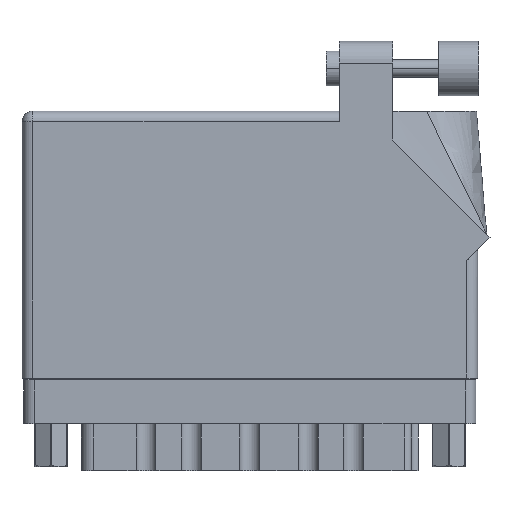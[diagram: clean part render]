
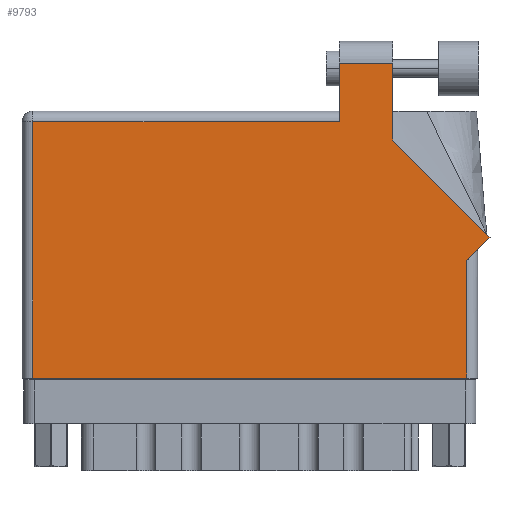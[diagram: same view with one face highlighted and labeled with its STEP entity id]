
A CAD part, front view. The second image highlights one B-rep face of the part: STEP entity #9793.
In plain terms, the highlighted face is planar.
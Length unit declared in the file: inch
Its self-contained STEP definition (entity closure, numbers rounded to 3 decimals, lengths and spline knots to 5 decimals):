
#339 = EDGE_CURVE ( 'NONE', #10485, #43581, #3423, .T. ) ;
#1990 = VERTEX_POINT ( 'NONE', #50898 ) ;
#2652 = CARTESIAN_POINT ( 'NONE',  ( 2.55, 0.675, 0. ) ) ;
#2788 = CARTESIAN_POINT ( 'NONE',  ( 2.68271, 0.80771, 0. ) ) ;
#3423 = LINE ( 'NONE', #22628, #28336 ) ;
#4869 = DIRECTION ( 'NONE',  ( 0., 1., 0. ) ) ;
#5986 = EDGE_CURVE ( 'NONE', #24299, #54785, #29102, .T. ) ;
#6192 = VECTOR ( 'NONE', #15545, 39.37008 ) ;
#6231 = CARTESIAN_POINT ( 'NONE',  ( 0.062, 0., 0. ) ) ;
#6344 = CARTESIAN_POINT ( 'NONE',  ( 2.126, 1.805, 0. ) ) ;
#7420 = LINE ( 'NONE', #25991, #21301 ) ;
#8194 = CARTESIAN_POINT ( 'NONE',  ( 2.55, 0., 0. ) ) ;
#9665 = EDGE_CURVE ( 'NONE', #24457, #12983, #50404, .T. ) ;
#9793 = ADVANCED_FACE ( 'NONE', ( #14433 ), #18517, .F. ) ;
#10485 = VERTEX_POINT ( 'NONE', #60340 ) ;
#10664 = ORIENTED_EDGE ( 'NONE', *, *, #339, .T. ) ;
#12126 = ORIENTED_EDGE ( 'NONE', *, *, #16217, .T. ) ;
#12679 = ORIENTED_EDGE ( 'NONE', *, *, #15060, .T. ) ;
#12983 = VERTEX_POINT ( 'NONE', #47654 ) ;
#14296 = LINE ( 'NONE', #19327, #6192 ) ;
#14376 = ORIENTED_EDGE ( 'NONE', *, *, #9665, .T. ) ;
#14433 = FACE_OUTER_BOUND ( 'NONE', #40207, .T. ) ;
#14602 = CARTESIAN_POINT ( 'NONE',  ( 1.819, 1.805, 0. ) ) ;
#14739 = DIRECTION ( 'NONE',  ( -0.707, 0.707, 0. ) ) ;
#15060 = EDGE_CURVE ( 'NONE', #43581, #24299, #20052, .T. ) ;
#15545 = DIRECTION ( 'NONE',  ( 0., 1., 0. ) ) ;
#16217 = EDGE_CURVE ( 'NONE', #1990, #30200, #33837, .T. ) ;
#17422 = EDGE_CURVE ( 'NONE', #54785, #24457, #42731, .T. ) ;
#18517 = PLANE ( 'NONE',  #32295 ) ;
#19327 = CARTESIAN_POINT ( 'NONE',  ( 2.126, 1.36442, 0. ) ) ;
#19530 = CARTESIAN_POINT ( 'NONE',  ( 2.68271, 0.80771, 0. ) ) ;
#20052 = LINE ( 'NONE', #34207, #56727 ) ;
#21301 = VECTOR ( 'NONE', #45898, 39.37008 ) ;
#22628 = CARTESIAN_POINT ( 'NONE',  ( 0.062, 0., 0. ) ) ;
#23240 = VECTOR ( 'NONE', #14739, 39.37008 ) ;
#23478 = DIRECTION ( 'NONE',  ( 0., -1., 0. ) ) ;
#24299 = VERTEX_POINT ( 'NONE', #8194 ) ;
#24457 = VERTEX_POINT ( 'NONE', #19530 ) ;
#25991 = CARTESIAN_POINT ( 'NONE',  ( 0., 1.468, 0. ) ) ;
#27640 = ORIENTED_EDGE ( 'NONE', *, *, #17422, .T. ) ;
#28336 = VECTOR ( 'NONE', #56695, 39.37008 ) ;
#29102 = LINE ( 'NONE', #51867, #45585 ) ;
#30200 = VERTEX_POINT ( 'NONE', #54878 ) ;
#31671 = DIRECTION ( 'NONE',  ( 0.707, 0.707, 0. ) ) ;
#32295 = AXIS2_PLACEMENT_3D ( 'NONE', #33605, #38680, #52894 ) ;
#32795 = EDGE_CURVE ( 'NONE', #30200, #10485, #7420, .T. ) ;
#33204 = CARTESIAN_POINT ( 'NONE',  ( 1.819, 1.53, 0. ) ) ;
#33605 = CARTESIAN_POINT ( 'NONE',  ( 0., 1.53, 0. ) ) ;
#33779 = DIRECTION ( 'NONE',  ( -1., 0., 0. ) ) ;
#33837 = LINE ( 'NONE', #33204, #48036 ) ;
#34207 = CARTESIAN_POINT ( 'NONE',  ( 0., 0., 0. ) ) ;
#37326 = ORIENTED_EDGE ( 'NONE', *, *, #60133, .T. ) ;
#38030 = DIRECTION ( 'NONE',  ( 1., 0., 0. ) ) ;
#38680 = DIRECTION ( 'NONE',  ( 0., 0., -1. ) ) ;
#40207 = EDGE_LOOP ( 'NONE', ( #62073, #37326, #12126, #54065, #10664, #12679, #47370, #27640, #14376 ) ) ;
#41800 = CARTESIAN_POINT ( 'NONE',  ( 2.612, 0.737, 0. ) ) ;
#42731 = LINE ( 'NONE', #41800, #49117 ) ;
#43581 = VERTEX_POINT ( 'NONE', #6231 ) ;
#45585 = VECTOR ( 'NONE', #4869, 39.37008 ) ;
#45898 = DIRECTION ( 'NONE',  ( -1., 0., 0. ) ) ;
#47370 = ORIENTED_EDGE ( 'NONE', *, *, #5986, .T. ) ;
#47448 = VERTEX_POINT ( 'NONE', #6344 ) ;
#47654 = CARTESIAN_POINT ( 'NONE',  ( 2.126, 1.36442, 0. ) ) ;
#48036 = VECTOR ( 'NONE', #23478, 39.37008 ) ;
#48444 = VECTOR ( 'NONE', #33779, 39.37008 ) ;
#49117 = VECTOR ( 'NONE', #31671, 39.37008 ) ;
#50404 = LINE ( 'NONE', #2788, #23240 ) ;
#50898 = CARTESIAN_POINT ( 'NONE',  ( 1.819, 1.805, 0. ) ) ;
#51867 = CARTESIAN_POINT ( 'NONE',  ( 2.55, 0.737, 0. ) ) ;
#52894 = DIRECTION ( 'NONE',  ( -1., 0., 0. ) ) ;
#54065 = ORIENTED_EDGE ( 'NONE', *, *, #32795, .T. ) ;
#54785 = VERTEX_POINT ( 'NONE', #2652 ) ;
#54878 = CARTESIAN_POINT ( 'NONE',  ( 1.819, 1.468, 0. ) ) ;
#56695 = DIRECTION ( 'NONE',  ( 0., -1., 0. ) ) ;
#56727 = VECTOR ( 'NONE', #38030, 39.37008 ) ;
#57811 = LINE ( 'NONE', #14602, #48444 ) ;
#60133 = EDGE_CURVE ( 'NONE', #47448, #1990, #57811, .T. ) ;
#60340 = CARTESIAN_POINT ( 'NONE',  ( 0.062, 1.468, 0. ) ) ;
#61464 = EDGE_CURVE ( 'NONE', #12983, #47448, #14296, .T. ) ;
#62073 = ORIENTED_EDGE ( 'NONE', *, *, #61464, .T. ) ;
